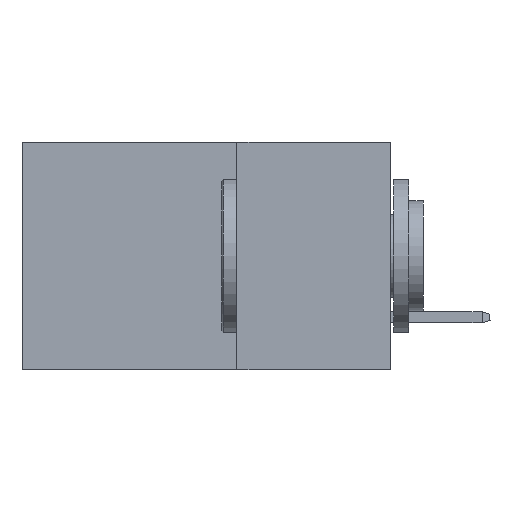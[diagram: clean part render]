
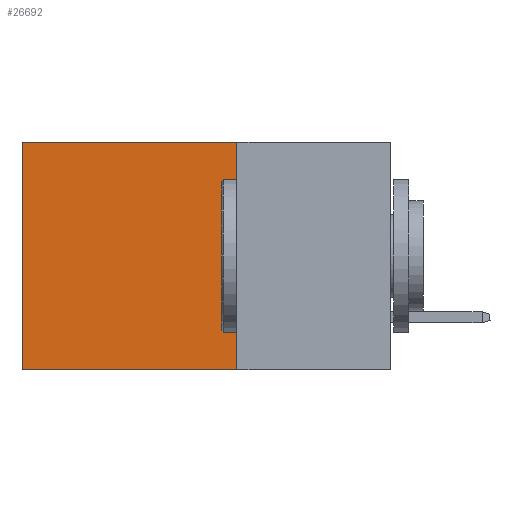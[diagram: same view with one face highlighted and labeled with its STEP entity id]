
A CAD part, left-side view. The second image highlights one B-rep face of the part: STEP entity #26692.
In plain terms, the highlighted planar face has unit normal (-1, 0, 0).
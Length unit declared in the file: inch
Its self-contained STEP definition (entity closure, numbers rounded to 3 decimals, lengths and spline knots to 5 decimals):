
#27 = VECTOR ( 'NONE', #20290, 39.37008 ) ;
#385 = EDGE_LOOP ( 'NONE', ( #18995, #27817, #639, #14261 ) ) ;
#639 = ORIENTED_EDGE ( 'NONE', *, *, #4494, .F. ) ;
#1333 = CARTESIAN_POINT ( 'NONE',  ( 0.2875, 0.6, -0.37 ) ) ;
#2769 = VECTOR ( 'NONE', #4799, 39.37008 ) ;
#3186 = DIRECTION ( 'NONE',  ( 1., 0., 0. ) ) ;
#3191 = FACE_OUTER_BOUND ( 'NONE', #385, .T. ) ;
#4494 = EDGE_CURVE ( 'NONE', #14685, #24687, #13735, .T. ) ;
#4799 = DIRECTION ( 'NONE',  ( 0., 1., 0. ) ) ;
#5734 = VECTOR ( 'NONE', #6575, 39.37008 ) ;
#5993 = VECTOR ( 'NONE', #18073, 39.37008 ) ;
#6384 = AXIS2_PLACEMENT_3D ( 'NONE', #16702, #3186, #23261 ) ;
#6575 = DIRECTION ( 'NONE',  ( 0., 1., 0. ) ) ;
#9254 = CARTESIAN_POINT ( 'NONE',  ( 0.2875, 0.25, -0.37 ) ) ;
#9597 = PLANE ( 'NONE',  #6384 ) ;
#11275 = VERTEX_POINT ( 'NONE', #15868 ) ;
#11377 = LINE ( 'NONE', #15923, #5734 ) ;
#11614 = LINE ( 'NONE', #22960, #2769 ) ;
#12380 = LINE ( 'NONE', #24930, #27 ) ;
#13735 = LINE ( 'NONE', #27148, #5993 ) ;
#14079 = EDGE_CURVE ( 'NONE', #14685, #11275, #11614, .T. ) ;
#14261 = ORIENTED_EDGE ( 'NONE', *, *, #14079, .T. ) ;
#14685 = VERTEX_POINT ( 'NONE', #17435 ) ;
#15868 = CARTESIAN_POINT ( 'NONE',  ( 0.2875, 0.6, 0. ) ) ;
#15923 = CARTESIAN_POINT ( 'NONE',  ( 0.2875, 0.25, -0.37 ) ) ;
#16702 = CARTESIAN_POINT ( 'NONE',  ( 0.2875, 0.25, 0. ) ) ;
#17435 = CARTESIAN_POINT ( 'NONE',  ( 0.2875, 0.25, 0. ) ) ;
#18073 = DIRECTION ( 'NONE',  ( 0., 0., -1. ) ) ;
#18995 = ORIENTED_EDGE ( 'NONE', *, *, #25774, .T. ) ;
#20290 = DIRECTION ( 'NONE',  ( 0., 0., -1. ) ) ;
#22382 = VERTEX_POINT ( 'NONE', #1333 ) ;
#22960 = CARTESIAN_POINT ( 'NONE',  ( 0.2875, 0.25, 0. ) ) ;
#23261 = DIRECTION ( 'NONE',  ( 0., 0., -1. ) ) ;
#24687 = VERTEX_POINT ( 'NONE', #9254 ) ;
#24930 = CARTESIAN_POINT ( 'NONE',  ( 0.2875, 0.6, 0. ) ) ;
#25225 = EDGE_CURVE ( 'NONE', #24687, #22382, #11377, .T. ) ;
#25774 = EDGE_CURVE ( 'NONE', #11275, #22382, #12380, .T. ) ;
#26692 = ADVANCED_FACE ( 'NONE', ( #3191 ), #9597, .F. ) ;
#27148 = CARTESIAN_POINT ( 'NONE',  ( 0.2875, 0.25, 0. ) ) ;
#27817 = ORIENTED_EDGE ( 'NONE', *, *, #25225, .F. ) ;
